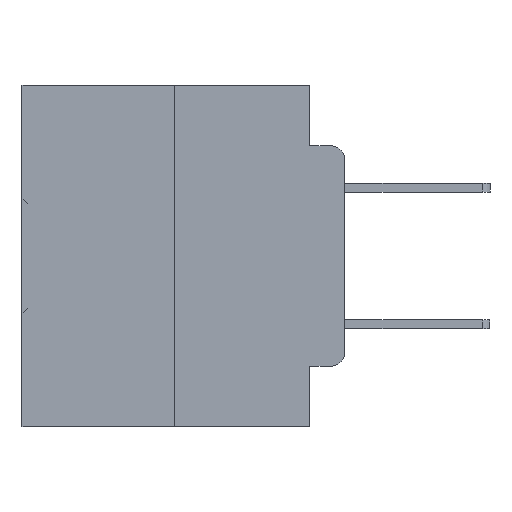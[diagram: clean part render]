
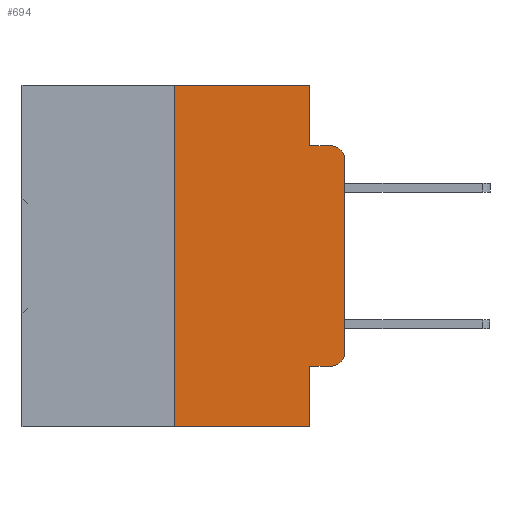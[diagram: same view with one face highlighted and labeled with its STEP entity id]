
A CAD part, left-side view. The second image highlights one B-rep face of the part: STEP entity #694.
In plain terms, the highlighted planar face has unit normal (-1, 0, 0).
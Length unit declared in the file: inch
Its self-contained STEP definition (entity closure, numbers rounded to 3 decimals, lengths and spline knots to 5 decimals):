
#39 = DIRECTION ( 'NONE',  ( 0., -1., 0. ) ) ;
#142 = CARTESIAN_POINT ( 'NONE',  ( 0., 0.051, 0. ) ) ;
#694 = ADVANCED_FACE ( 'NONE', ( #22062 ), #4841, .F. ) ;
#1036 = CARTESIAN_POINT ( 'NONE',  ( 0., 0.02, -0.1085 ) ) ;
#1202 = CARTESIAN_POINT ( 'NONE',  ( 0., 0.473, 0. ) ) ;
#1648 = LINE ( 'NONE', #2682, #8972 ) ;
#2572 = CARTESIAN_POINT ( 'NONE',  ( 0., 0.051, -0.4115 ) ) ;
#2682 = CARTESIAN_POINT ( 'NONE',  ( 0., 0., 0. ) ) ;
#2937 = DIRECTION ( 'NONE',  ( 0., 0., -1. ) ) ;
#3483 = CARTESIAN_POINT ( 'NONE',  ( 0., 0., -0.3915 ) ) ;
#3705 = VERTEX_POINT ( 'NONE', #8909 ) ;
#3800 = DIRECTION ( 'NONE',  ( 0., 0., -1. ) ) ;
#3827 = ORIENTED_EDGE ( 'NONE', *, *, #34152, .T. ) ;
#3941 = VERTEX_POINT ( 'NONE', #4632 ) ;
#3968 = VERTEX_POINT ( 'NONE', #21283 ) ;
#4078 = DIRECTION ( 'NONE',  ( 0., -1., 0. ) ) ;
#4155 = DIRECTION ( 'NONE',  ( 0., -1., 0. ) ) ;
#4365 = ORIENTED_EDGE ( 'NONE', *, *, #16310, .T. ) ;
#4632 = CARTESIAN_POINT ( 'NONE',  ( 0., 0.051, -0.0885 ) ) ;
#4737 = DIRECTION ( 'NONE',  ( 1., 0., 0. ) ) ;
#4769 = ORIENTED_EDGE ( 'NONE', *, *, #16767, .F. ) ;
#4841 = PLANE ( 'NONE',  #9187 ) ;
#5154 = ORIENTED_EDGE ( 'NONE', *, *, #14444, .F. ) ;
#5674 = ORIENTED_EDGE ( 'NONE', *, *, #8751, .F. ) ;
#6705 = ORIENTED_EDGE ( 'NONE', *, *, #26106, .F. ) ;
#7038 = ORIENTED_EDGE ( 'NONE', *, *, #31933, .T. ) ;
#7117 = ORIENTED_EDGE ( 'NONE', *, *, #31053, .F. ) ;
#7467 = ORIENTED_EDGE ( 'NONE', *, *, #33421, .T. ) ;
#7727 = DIRECTION ( 'NONE',  ( -1., 0., 0. ) ) ;
#7786 = ORIENTED_EDGE ( 'NONE', *, *, #22859, .T. ) ;
#8748 = CARTESIAN_POINT ( 'NONE',  ( 0., 0.25, 0. ) ) ;
#8751 = EDGE_CURVE ( 'NONE', #22333, #23239, #18290, .T. ) ;
#8909 = CARTESIAN_POINT ( 'NONE',  ( 0., 0.051, -0.5 ) ) ;
#8972 = VECTOR ( 'NONE', #32521, 39.37008 ) ;
#9187 = AXIS2_PLACEMENT_3D ( 'NONE', #20922, #4737, #9669 ) ;
#9296 = LINE ( 'NONE', #8748, #23066 ) ;
#9486 = CARTESIAN_POINT ( 'NONE',  ( 0., 0.473, -0.5 ) ) ;
#9669 = DIRECTION ( 'NONE',  ( 0., 0., -1. ) ) ;
#10269 = CARTESIAN_POINT ( 'NONE',  ( 0., 0.02, -0.4115 ) ) ;
#10285 = VECTOR ( 'NONE', #39, 39.37008 ) ;
#12685 = CARTESIAN_POINT ( 'NONE',  ( 0., 0., -0.1085 ) ) ;
#13766 = VECTOR ( 'NONE', #23985, 39.37008 ) ;
#13891 = VERTEX_POINT ( 'NONE', #2572 ) ;
#14227 = CIRCLE ( 'NONE', #18108, 0.02 ) ;
#14444 = EDGE_CURVE ( 'NONE', #23239, #3941, #14764, .T. ) ;
#14644 = LINE ( 'NONE', #29166, #13766 ) ;
#14764 = LINE ( 'NONE', #34541, #20359 ) ;
#16310 = EDGE_CURVE ( 'NONE', #16488, #17865, #24897, .T. ) ;
#16488 = VERTEX_POINT ( 'NONE', #12685 ) ;
#16767 = EDGE_CURVE ( 'NONE', #3941, #17865, #18463, .T. ) ;
#17865 = VERTEX_POINT ( 'NONE', #21774 ) ;
#18104 = LINE ( 'NONE', #9486, #27438 ) ;
#18108 = AXIS2_PLACEMENT_3D ( 'NONE', #24179, #7727, #26843 ) ;
#18290 = LINE ( 'NONE', #1202, #24703 ) ;
#18463 = LINE ( 'NONE', #29954, #10285 ) ;
#19033 = LINE ( 'NONE', #142, #27072 ) ;
#20309 = DIRECTION ( 'NONE',  ( -1., 0., 0. ) ) ;
#20359 = VECTOR ( 'NONE', #21425, 39.37008 ) ;
#20922 = CARTESIAN_POINT ( 'NONE',  ( 0., 0.473, 0. ) ) ;
#21283 = CARTESIAN_POINT ( 'NONE',  ( 0., 0.25, -0.5 ) ) ;
#21425 = DIRECTION ( 'NONE',  ( 0., 0., -1. ) ) ;
#21774 = CARTESIAN_POINT ( 'NONE',  ( 0., 0.02, -0.0885 ) ) ;
#22062 = FACE_OUTER_BOUND ( 'NONE', #26305, .T. ) ;
#22333 = VERTEX_POINT ( 'NONE', #27434 ) ;
#22859 = EDGE_CURVE ( 'NONE', #34004, #31780, #14227, .T. ) ;
#23066 = VECTOR ( 'NONE', #30440, 39.37008 ) ;
#23239 = VERTEX_POINT ( 'NONE', #23694 ) ;
#23694 = CARTESIAN_POINT ( 'NONE',  ( 0., 0.051, 0. ) ) ;
#23985 = DIRECTION ( 'NONE',  ( 0., -1., 0. ) ) ;
#24179 = CARTESIAN_POINT ( 'NONE',  ( 0., 0.02, -0.3915 ) ) ;
#24703 = VECTOR ( 'NONE', #4078, 39.37008 ) ;
#24897 = CIRCLE ( 'NONE', #26845, 0.02 ) ;
#26106 = EDGE_CURVE ( 'NONE', #3968, #22333, #9296, .T. ) ;
#26305 = EDGE_LOOP ( 'NONE', ( #3827, #4365, #4769, #5154, #5674, #6705, #7038, #7117, #7467, #7786 ) ) ;
#26843 = DIRECTION ( 'NONE',  ( 0., 0., -1. ) ) ;
#26845 = AXIS2_PLACEMENT_3D ( 'NONE', #1036, #20309, #3800 ) ;
#27072 = VECTOR ( 'NONE', #2937, 39.37008 ) ;
#27434 = CARTESIAN_POINT ( 'NONE',  ( 0., 0.25, 0. ) ) ;
#27438 = VECTOR ( 'NONE', #4155, 39.37008 ) ;
#29166 = CARTESIAN_POINT ( 'NONE',  ( 0., 0.051, -0.4115 ) ) ;
#29954 = CARTESIAN_POINT ( 'NONE',  ( 0., 0.051, -0.0885 ) ) ;
#30440 = DIRECTION ( 'NONE',  ( 0., 0., 1. ) ) ;
#31053 = EDGE_CURVE ( 'NONE', #13891, #3705, #19033, .T. ) ;
#31780 = VERTEX_POINT ( 'NONE', #3483 ) ;
#31933 = EDGE_CURVE ( 'NONE', #3968, #3705, #18104, .T. ) ;
#32521 = DIRECTION ( 'NONE',  ( 0., 0., 1. ) ) ;
#33421 = EDGE_CURVE ( 'NONE', #13891, #34004, #14644, .T. ) ;
#34004 = VERTEX_POINT ( 'NONE', #10269 ) ;
#34152 = EDGE_CURVE ( 'NONE', #31780, #16488, #1648, .T. ) ;
#34541 = CARTESIAN_POINT ( 'NONE',  ( 0., 0.051, 0. ) ) ;
